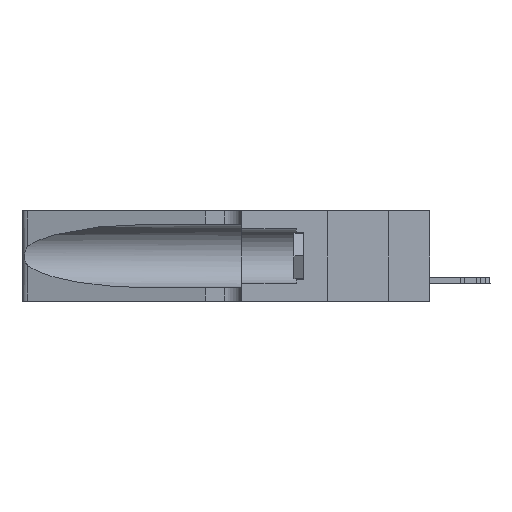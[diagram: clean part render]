
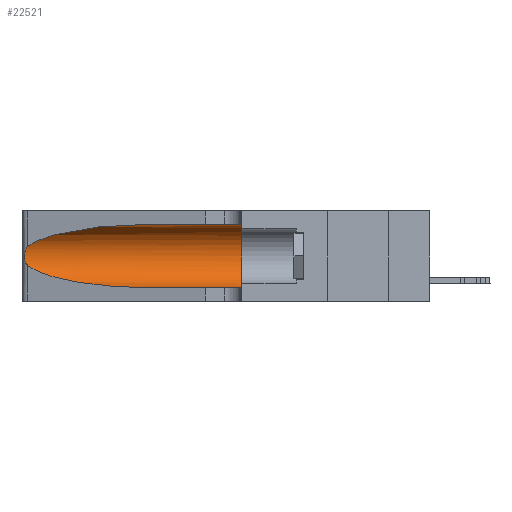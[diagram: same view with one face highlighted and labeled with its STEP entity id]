
A CAD part, left-side view. The second image highlights one B-rep face of the part: STEP entity #22521.
In plain terms, the highlighted cylindrical face has radius 3.308 mm (diameter 6.617 mm), a partial arc.
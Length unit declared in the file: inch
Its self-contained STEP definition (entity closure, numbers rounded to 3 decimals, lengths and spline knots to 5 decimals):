
#206 = ORIENTED_EDGE ( 'NONE', *, *, #22450, .T. ) ;
#1376 = VERTEX_POINT ( 'NONE', #26310 ) ;
#2130 = CARTESIAN_POINT ( 'NONE',  ( 0.1305, 0.35, 0.05475 ) ) ;
#2813 = CARTESIAN_POINT ( 'NONE',  ( 0.25854, 1.2359, 0.20912 ) ) ;
#3139 = CARTESIAN_POINT ( 'NONE',  ( 0.1305, 0.72297, 0.31525 ) ) ;
#3785 = CARTESIAN_POINT ( 'NONE',  ( 0.25856, 1.23593, 0.16098 ) ) ;
#4405 = VECTOR ( 'NONE', #30647, 39.37008 ) ;
#5714 = DIRECTION ( 'NONE',  ( 0., -1., 0. ) ) ;
#5968 = ORIENTED_EDGE ( 'NONE', *, *, #26228, .T. ) ;
#6844 = DIRECTION ( 'NONE',  ( 0., 1., 0. ) ) ;
#7363 = CARTESIAN_POINT ( 'NONE',  ( 0.25639, 1.23184, 0.21858 ) ) ;
#8715 = CARTESIAN_POINT ( 'NONE',  ( 0.25639, 1.23186, 0.15144 ) ) ;
#10413 = FACE_OUTER_BOUND ( 'NONE', #32556, .T. ) ;
#12205 = CARTESIAN_POINT ( 'NONE',  ( 0.25487, 1.22718, 0.14631 ) ) ;
#12212 = CARTESIAN_POINT ( 'NONE',  ( 0.25789, 1.23486, 0.15765 ) ) ;
#12309 = ORIENTED_EDGE ( 'NONE', *, *, #12760, .T. ) ;
#12442 = CARTESIAN_POINT ( 'NONE',  ( 0.25487, 1.22718, 0.14631 ) ) ;
#12760 = EDGE_CURVE ( 'NONE', #34939, #40910, #22018, .T. ) ;
#14068 = VERTEX_POINT ( 'NONE', #12205 ) ;
#15566 = B_SPLINE_CURVE_WITH_KNOTS ( 'NONE', 3,
 ( #20907, #46784, #7363, #29181, #2813, #30424, #31680, #23328, #23430, #3785, #12212, #8715, #37683, #12442 ),
 .UNSPECIFIED., .F., .F.,
 ( 4, 2, 2, 2, 2, 2, 4 ),
 ( 0., 0.00027, 0.00053, 0.00107, 0.0016, 0.00187, 0.00214 ),
 .UNSPECIFIED. ) ;
#20907 = CARTESIAN_POINT ( 'NONE',  ( 0.25487, 1.22718, 0.22369 ) ) ;
#21170 =( BOUNDED_CURVE ( )  B_SPLINE_CURVE ( 3, ( #41889, #41401, #31428, #28272 ),
 .UNSPECIFIED., .F., .F. ) 
 B_SPLINE_CURVE_WITH_KNOTS ( ( 4, 4 ),
 ( 3.44316, 4.71239 ),
 .UNSPECIFIED. ) 
 CURVE ( )  GEOMETRIC_REPRESENTATION_ITEM ( )  RATIONAL_B_SPLINE_CURVE ( ( 1., 0.87, 0.87, 1. ) ) 
 REPRESENTATION_ITEM ( '' )  );
#21591 = DIRECTION ( 'NONE',  ( 0., 0., 1. ) ) ;
#22018 = LINE ( 'NONE', #26689, #4405 ) ;
#22450 = EDGE_CURVE ( 'NONE', #44830, #14068, #15566, .T. ) ;
#22521 = ADVANCED_FACE ( 'NONE', ( #10413 ), #42592, .F. ) ;
#23015 = CARTESIAN_POINT ( 'NONE',  ( 0.1305, 1.61858, 0.31525 ) ) ;
#23170 = EDGE_CURVE ( 'NONE', #46485, #1376, #27064, .T. ) ;
#23328 = CARTESIAN_POINT ( 'NONE',  ( 0.26075, 1.23896, 0.178 ) ) ;
#23430 = CARTESIAN_POINT ( 'NONE',  ( 0.26017, 1.23833, 0.17102 ) ) ;
#23693 = VECTOR ( 'NONE', #30260, 39.37008 ) ;
#25688 = EDGE_CURVE ( 'NONE', #1376, #40910, #32515, .T. ) ;
#26228 = EDGE_CURVE ( 'NONE', #14068, #34939, #21170, .T. ) ;
#26310 = CARTESIAN_POINT ( 'NONE',  ( 0.1305, 0.35, 0.31525 ) ) ;
#26689 = CARTESIAN_POINT ( 'NONE',  ( 0.1305, 1.61858, 0.05475 ) ) ;
#27064 = LINE ( 'NONE', #23015, #23693 ) ;
#27139 = CARTESIAN_POINT ( 'NONE',  ( 0.2373, 1.15595, 0.28018 ) ) ;
#28272 = CARTESIAN_POINT ( 'NONE',  ( 0.1305, 0.72297, 0.05475 ) ) ;
#28751 = DIRECTION ( 'NONE',  ( 0., 0., -1. ) ) ;
#29181 = CARTESIAN_POINT ( 'NONE',  ( 0.25787, 1.23484, 0.2124 ) ) ;
#30215 = CARTESIAN_POINT ( 'NONE',  ( 0.1305, 0.72297, 0.05475 ) ) ;
#30260 = DIRECTION ( 'NONE',  ( 0., -1., 0. ) ) ;
#30424 = CARTESIAN_POINT ( 'NONE',  ( 0.26018, 1.23835, 0.19895 ) ) ;
#30647 = DIRECTION ( 'NONE',  ( 0., -1., 0. ) ) ;
#31380 = AXIS2_PLACEMENT_3D ( 'NONE', #37711, #5714, #28751 ) ;
#31428 = CARTESIAN_POINT ( 'NONE',  ( 0.18966, 0.96281, 0.05475 ) ) ;
#31680 = CARTESIAN_POINT ( 'NONE',  ( 0.26075, 1.23896, 0.19203 ) ) ;
#32229 = ORIENTED_EDGE ( 'NONE', *, *, #23170, .F. ) ;
#32515 = CIRCLE ( 'NONE', #37795, 0.13025 ) ;
#32556 = EDGE_LOOP ( 'NONE', ( #41094, #206, #5968, #12309, #40705, #32229 ) ) ;
#34268 = CARTESIAN_POINT ( 'NONE',  ( 0.25487, 1.22718, 0.22369 ) ) ;
#34703 = EDGE_CURVE ( 'NONE', #46485, #44830, #35977, .T. ) ;
#34939 = VERTEX_POINT ( 'NONE', #30215 ) ;
#35977 =( BOUNDED_CURVE ( )  B_SPLINE_CURVE ( 3, ( #3139, #46325, #27139, #34268 ),
 .UNSPECIFIED., .F., .F. ) 
 B_SPLINE_CURVE_WITH_KNOTS ( ( 4, 4 ),
 ( 1.5708, 2.84003 ),
 .UNSPECIFIED. ) 
 CURVE ( )  GEOMETRIC_REPRESENTATION_ITEM ( )  RATIONAL_B_SPLINE_CURVE ( ( 1., 0.87, 0.87, 1. ) ) 
 REPRESENTATION_ITEM ( '' )  );
#37159 = CARTESIAN_POINT ( 'NONE',  ( 0.25487, 1.22718, 0.22369 ) ) ;
#37683 = CARTESIAN_POINT ( 'NONE',  ( 0.25555, 1.22993, 0.14849 ) ) ;
#37711 = CARTESIAN_POINT ( 'NONE',  ( 0.1305, 1.61858, 0.185 ) ) ;
#37795 = AXIS2_PLACEMENT_3D ( 'NONE', #39444, #6844, #21591 ) ;
#39444 = CARTESIAN_POINT ( 'NONE',  ( 0.1305, 0.35, 0.185 ) ) ;
#40705 = ORIENTED_EDGE ( 'NONE', *, *, #25688, .F. ) ;
#40910 = VERTEX_POINT ( 'NONE', #2130 ) ;
#41094 = ORIENTED_EDGE ( 'NONE', *, *, #34703, .T. ) ;
#41401 = CARTESIAN_POINT ( 'NONE',  ( 0.2373, 1.15595, 0.08982 ) ) ;
#41889 = CARTESIAN_POINT ( 'NONE',  ( 0.25487, 1.22718, 0.14631 ) ) ;
#42592 = CYLINDRICAL_SURFACE ( 'NONE', #31380, 0.13025 ) ;
#42808 = CARTESIAN_POINT ( 'NONE',  ( 0.1305, 0.72297, 0.31525 ) ) ;
#44830 = VERTEX_POINT ( 'NONE', #37159 ) ;
#46325 = CARTESIAN_POINT ( 'NONE',  ( 0.18966, 0.96281, 0.31525 ) ) ;
#46485 = VERTEX_POINT ( 'NONE', #42808 ) ;
#46784 = CARTESIAN_POINT ( 'NONE',  ( 0.25555, 1.22994, 0.2215 ) ) ;
